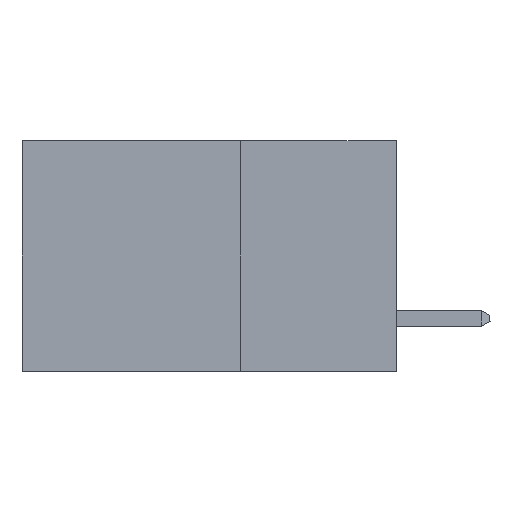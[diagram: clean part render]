
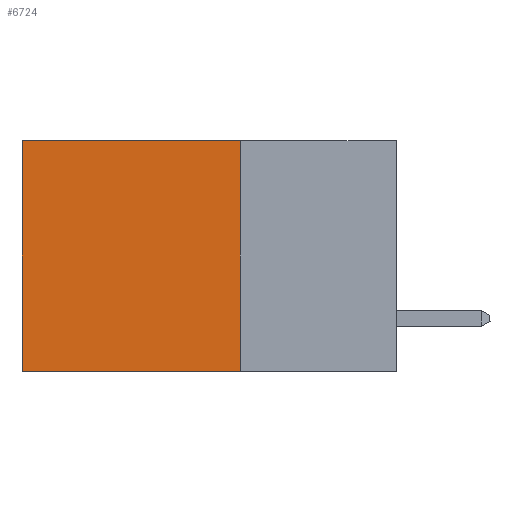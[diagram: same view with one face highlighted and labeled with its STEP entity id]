
A CAD part, left-side view. The second image highlights one B-rep face of the part: STEP entity #6724.
In plain terms, the highlighted planar face has unit normal (-1, 0, 0).
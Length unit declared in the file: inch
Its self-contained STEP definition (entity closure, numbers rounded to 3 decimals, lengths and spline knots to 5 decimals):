
#1543 = EDGE_CURVE ( 'NONE', #1649, #3930, #10713, .T. ) ;
#1590 = AXIS2_PLACEMENT_3D ( 'NONE', #12729, #12572, #12555 ) ;
#1649 = VERTEX_POINT ( 'NONE', #9393 ) ;
#1708 = VERTEX_POINT ( 'NONE', #9689 ) ;
#1761 = VECTOR ( 'NONE', #12497, 39.37008 ) ;
#2365 = ORIENTED_EDGE ( 'NONE', *, *, #10330, .F. ) ;
#2458 = LINE ( 'NONE', #3437, #13892 ) ;
#2765 = LINE ( 'NONE', #14225, #5760 ) ;
#3177 = DIRECTION ( 'NONE',  ( 0., 0., -1. ) ) ;
#3235 = EDGE_CURVE ( 'NONE', #1708, #4837, #2765, .T. ) ;
#3329 = DIRECTION ( 'NONE',  ( 0., 0., -1. ) ) ;
#3437 = CARTESIAN_POINT ( 'NONE',  ( 0.298, 0.6, 0. ) ) ;
#3761 = EDGE_LOOP ( 'NONE', ( #5061, #10914, #2365, #8356 ) ) ;
#3930 = VERTEX_POINT ( 'NONE', #3991 ) ;
#3991 = CARTESIAN_POINT ( 'NONE',  ( 0.298, 0.6, 0. ) ) ;
#4837 = VERTEX_POINT ( 'NONE', #5240 ) ;
#5061 = ORIENTED_EDGE ( 'NONE', *, *, #7433, .T. ) ;
#5240 = CARTESIAN_POINT ( 'NONE',  ( 0.298, 0.6, -0.37 ) ) ;
#5760 = VECTOR ( 'NONE', #13754, 39.37008 ) ;
#6724 = ADVANCED_FACE ( 'NONE', ( #8645 ), #12595, .F. ) ;
#7433 = EDGE_CURVE ( 'NONE', #3930, #4837, #2458, .T. ) ;
#7705 = CARTESIAN_POINT ( 'NONE',  ( 0.298, 0.25, 0. ) ) ;
#8356 = ORIENTED_EDGE ( 'NONE', *, *, #1543, .T. ) ;
#8645 = FACE_OUTER_BOUND ( 'NONE', #3761, .T. ) ;
#9393 = CARTESIAN_POINT ( 'NONE',  ( 0.298, 0.25, 0. ) ) ;
#9689 = CARTESIAN_POINT ( 'NONE',  ( 0.298, 0.25, -0.37 ) ) ;
#9990 = CARTESIAN_POINT ( 'NONE',  ( 0.298, 0.25, 0. ) ) ;
#10330 = EDGE_CURVE ( 'NONE', #1649, #1708, #11046, .T. ) ;
#10687 = VECTOR ( 'NONE', #3329, 39.37008 ) ;
#10713 = LINE ( 'NONE', #7705, #1761 ) ;
#10914 = ORIENTED_EDGE ( 'NONE', *, *, #3235, .F. ) ;
#11046 = LINE ( 'NONE', #9990, #10687 ) ;
#12497 = DIRECTION ( 'NONE',  ( 0., 1., 0. ) ) ;
#12555 = DIRECTION ( 'NONE',  ( 0., 0., -1. ) ) ;
#12572 = DIRECTION ( 'NONE',  ( 1., 0., 0. ) ) ;
#12595 = PLANE ( 'NONE',  #1590 ) ;
#12729 = CARTESIAN_POINT ( 'NONE',  ( 0.298, 0.25, 0. ) ) ;
#13754 = DIRECTION ( 'NONE',  ( 0., 1., 0. ) ) ;
#13892 = VECTOR ( 'NONE', #3177, 39.37008 ) ;
#14225 = CARTESIAN_POINT ( 'NONE',  ( 0.298, 0.25, -0.37 ) ) ;
